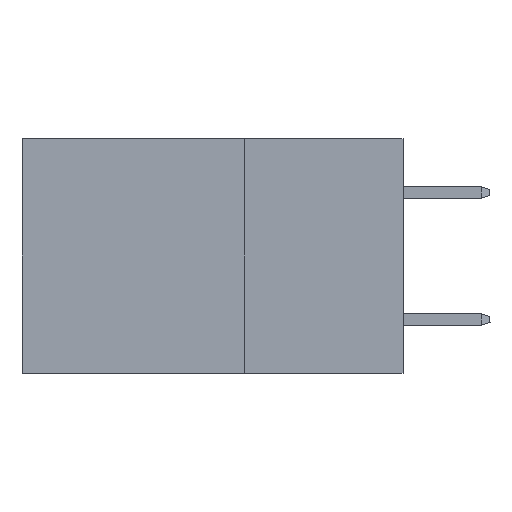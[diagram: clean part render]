
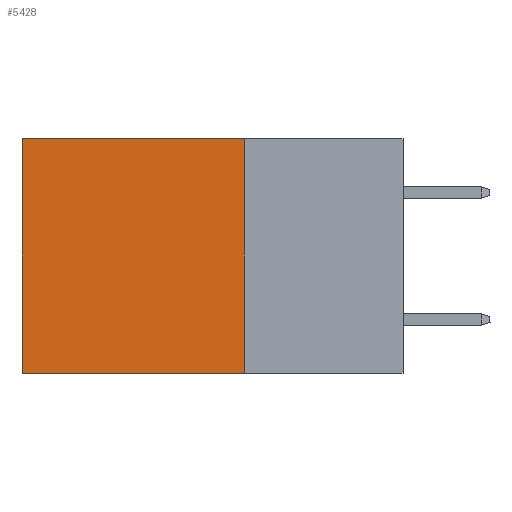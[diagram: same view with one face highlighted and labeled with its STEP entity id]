
A CAD part, left-side view. The second image highlights one B-rep face of the part: STEP entity #5428.
In plain terms, the highlighted planar face has unit normal (-1, 0, 0).
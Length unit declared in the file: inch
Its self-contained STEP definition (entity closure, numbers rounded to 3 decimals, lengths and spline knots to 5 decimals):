
#1130 = ORIENTED_EDGE ( 'NONE', *, *, #17497, .F. ) ;
#1275 = VECTOR ( 'NONE', #7177, 39.37008 ) ;
#1351 = LINE ( 'NONE', #4384, #1275 ) ;
#1972 = DIRECTION ( 'NONE',  ( 0., 0., -1. ) ) ;
#2165 = ORIENTED_EDGE ( 'NONE', *, *, #15969, .F. ) ;
#3304 = DIRECTION ( 'NONE',  ( 1., 0., 0. ) ) ;
#3516 = ORIENTED_EDGE ( 'NONE', *, *, #13810, .T. ) ;
#4302 = VERTEX_POINT ( 'NONE', #13155 ) ;
#4384 = CARTESIAN_POINT ( 'NONE',  ( 0.2875, 0.6, 0. ) ) ;
#5090 = CARTESIAN_POINT ( 'NONE',  ( 0.2875, 0.25, -0.37 ) ) ;
#5205 = VECTOR ( 'NONE', #13766, 39.37008 ) ;
#5428 = ADVANCED_FACE ( 'NONE', ( #7897 ), #16218, .F. ) ;
#5459 = VECTOR ( 'NONE', #11685, 39.37008 ) ;
#6023 = LINE ( 'NONE', #13277, #5459 ) ;
#6439 = VERTEX_POINT ( 'NONE', #16508 ) ;
#6519 = LINE ( 'NONE', #5090, #5205 ) ;
#7177 = DIRECTION ( 'NONE',  ( 0., 0., -1. ) ) ;
#7486 = VECTOR ( 'NONE', #7636, 39.37008 ) ;
#7636 = DIRECTION ( 'NONE',  ( 0., 1., 0. ) ) ;
#7793 = EDGE_LOOP ( 'NONE', ( #10095, #2165, #1130, #3516 ) ) ;
#7897 = FACE_OUTER_BOUND ( 'NONE', #7793, .T. ) ;
#8584 = VERTEX_POINT ( 'NONE', #14872 ) ;
#10095 = ORIENTED_EDGE ( 'NONE', *, *, #15656, .T. ) ;
#11685 = DIRECTION ( 'NONE',  ( 0., 0., -1. ) ) ;
#13155 = CARTESIAN_POINT ( 'NONE',  ( 0.2875, 0.25, 0. ) ) ;
#13277 = CARTESIAN_POINT ( 'NONE',  ( 0.2875, 0.25, 0. ) ) ;
#13566 = CARTESIAN_POINT ( 'NONE',  ( 0.2875, 0.25, 0. ) ) ;
#13689 = LINE ( 'NONE', #16433, #7486 ) ;
#13766 = DIRECTION ( 'NONE',  ( 0., 1., 0. ) ) ;
#13810 = EDGE_CURVE ( 'NONE', #4302, #8584, #13689, .T. ) ;
#14411 = CARTESIAN_POINT ( 'NONE',  ( 0.2875, 0.25, -0.37 ) ) ;
#14780 = VERTEX_POINT ( 'NONE', #14411 ) ;
#14872 = CARTESIAN_POINT ( 'NONE',  ( 0.2875, 0.6, 0. ) ) ;
#15140 = AXIS2_PLACEMENT_3D ( 'NONE', #13566, #3304, #1972 ) ;
#15656 = EDGE_CURVE ( 'NONE', #8584, #6439, #1351, .T. ) ;
#15969 = EDGE_CURVE ( 'NONE', #14780, #6439, #6519, .T. ) ;
#16218 = PLANE ( 'NONE',  #15140 ) ;
#16433 = CARTESIAN_POINT ( 'NONE',  ( 0.2875, 0.25, 0. ) ) ;
#16508 = CARTESIAN_POINT ( 'NONE',  ( 0.2875, 0.6, -0.37 ) ) ;
#17497 = EDGE_CURVE ( 'NONE', #4302, #14780, #6023, .T. ) ;
